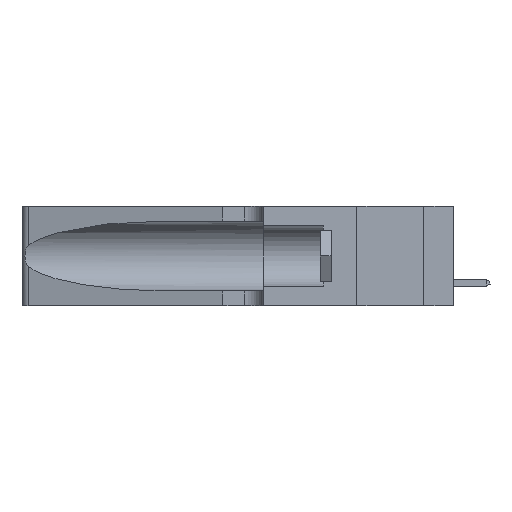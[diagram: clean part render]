
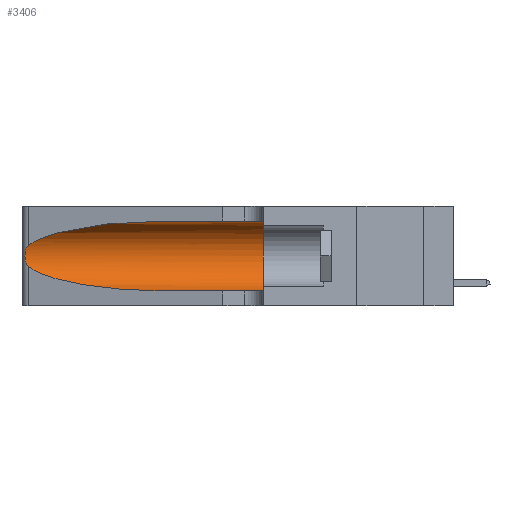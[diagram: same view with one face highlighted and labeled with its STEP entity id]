
A CAD part, left-side view. The second image highlights one B-rep face of the part: STEP entity #3406.
In plain terms, the highlighted cylindrical face has radius 3.308 mm (diameter 6.617 mm), a partial arc.
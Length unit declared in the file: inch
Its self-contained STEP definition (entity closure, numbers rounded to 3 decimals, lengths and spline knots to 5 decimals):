
#773 = DIRECTION ( 'NONE',  ( 0., 0., -1. ) ) ;
#1287 = CARTESIAN_POINT ( 'NONE',  ( 0.1305, 1.61858, 0.185 ) ) ;
#1504 = DIRECTION ( 'NONE',  ( 0., 1., 0. ) ) ;
#1772 = ORIENTED_EDGE ( 'NONE', *, *, #36571, .T. ) ;
#2330 = EDGE_CURVE ( 'NONE', #11419, #4882, #37015, .T. ) ;
#2530 = CARTESIAN_POINT ( 'NONE',  ( 0.25787, 1.23484, 0.2124 ) ) ;
#3406 = ADVANCED_FACE ( 'NONE', ( #35059 ), #34391, .F. ) ;
#4882 = VERTEX_POINT ( 'NONE', #51084 ) ;
#5034 = AXIS2_PLACEMENT_3D ( 'NONE', #48932, #1504, #29259 ) ;
#5925 = LINE ( 'NONE', #24997, #35693 ) ;
#5954 = CARTESIAN_POINT ( 'NONE',  ( 0.1305, 0.35, 0.05475 ) ) ;
#6724 = CIRCLE ( 'NONE', #5034, 0.13025 ) ;
#6942 = CARTESIAN_POINT ( 'NONE',  ( 0.25789, 1.23486, 0.15765 ) ) ;
#7525 = ORIENTED_EDGE ( 'NONE', *, *, #16669, .T. ) ;
#8419 = VERTEX_POINT ( 'NONE', #15291 ) ;
#8648 = CARTESIAN_POINT ( 'NONE',  ( 0.2373, 1.15595, 0.28018 ) ) ;
#9358 = VERTEX_POINT ( 'NONE', #5954 ) ;
#10707 = CARTESIAN_POINT ( 'NONE',  ( 0.26075, 1.23896, 0.19203 ) ) ;
#11419 = VERTEX_POINT ( 'NONE', #11508 ) ;
#11508 = CARTESIAN_POINT ( 'NONE',  ( 0.1305, 0.72297, 0.31525 ) ) ;
#11758 = CARTESIAN_POINT ( 'NONE',  ( 0.1305, 0.72297, 0.05475 ) ) ;
#12000 = VECTOR ( 'NONE', #46282, 39.37008 ) ;
#13221 = EDGE_CURVE ( 'NONE', #18733, #9358, #5925, .T. ) ;
#15284 = CARTESIAN_POINT ( 'NONE',  ( 0.18966, 0.96281, 0.05475 ) ) ;
#15291 = CARTESIAN_POINT ( 'NONE',  ( 0.25487, 1.22718, 0.14631 ) ) ;
#16669 = EDGE_CURVE ( 'NONE', #4882, #8419, #50766, .T. ) ;
#17367 = EDGE_CURVE ( 'NONE', #23731, #9358, #6724, .T. ) ;
#18733 = VERTEX_POINT ( 'NONE', #11758 ) ;
#20065 = CARTESIAN_POINT ( 'NONE',  ( 0.1305, 1.61858, 0.31525 ) ) ;
#22287 = CARTESIAN_POINT ( 'NONE',  ( 0.25639, 1.23184, 0.21858 ) ) ;
#22631 = CARTESIAN_POINT ( 'NONE',  ( 0.26075, 1.23896, 0.178 ) ) ;
#23715 = ORIENTED_EDGE ( 'NONE', *, *, #2330, .T. ) ;
#23731 = VERTEX_POINT ( 'NONE', #34816 ) ;
#24167 = ORIENTED_EDGE ( 'NONE', *, *, #13221, .T. ) ;
#24209 = CARTESIAN_POINT ( 'NONE',  ( 0.18966, 0.96281, 0.31525 ) ) ;
#24997 = CARTESIAN_POINT ( 'NONE',  ( 0.1305, 1.61858, 0.05475 ) ) ;
#26633 = CARTESIAN_POINT ( 'NONE',  ( 0.25856, 1.23593, 0.16098 ) ) ;
#29259 = DIRECTION ( 'NONE',  ( 0., 0., 1. ) ) ;
#29900 = DIRECTION ( 'NONE',  ( 0., -1., 0. ) ) ;
#30049 = CARTESIAN_POINT ( 'NONE',  ( 0.25487, 1.22718, 0.22369 ) ) ;
#30255 = CARTESIAN_POINT ( 'NONE',  ( 0.25854, 1.2359, 0.20912 ) ) ;
#32325 = EDGE_CURVE ( 'NONE', #11419, #23731, #47311, .T. ) ;
#32343 = CARTESIAN_POINT ( 'NONE',  ( 0.1305, 0.72297, 0.31525 ) ) ;
#33664 = CARTESIAN_POINT ( 'NONE',  ( 0.25555, 1.22994, 0.2215 ) ) ;
#34219 = CARTESIAN_POINT ( 'NONE',  ( 0.26018, 1.23835, 0.19895 ) ) ;
#34265 = CARTESIAN_POINT ( 'NONE',  ( 0.25555, 1.22993, 0.14849 ) ) ;
#34391 = CYLINDRICAL_SURFACE ( 'NONE', #40762, 0.13025 ) ;
#34816 = CARTESIAN_POINT ( 'NONE',  ( 0.1305, 0.35, 0.31525 ) ) ;
#34830 = CARTESIAN_POINT ( 'NONE',  ( 0.2373, 1.15595, 0.08982 ) ) ;
#35059 = FACE_OUTER_BOUND ( 'NONE', #51047, .T. ) ;
#35349 = CARTESIAN_POINT ( 'NONE',  ( 0.25487, 1.22718, 0.14631 ) ) ;
#35693 = VECTOR ( 'NONE', #29900, 39.37008 ) ;
#36571 = EDGE_CURVE ( 'NONE', #8419, #18733, #43451, .T. ) ;
#36674 = DIRECTION ( 'NONE',  ( 0., -1., 0. ) ) ;
#37015 =( BOUNDED_CURVE ( )  B_SPLINE_CURVE ( 3, ( #32343, #24209, #8648, #47775 ),
 .UNSPECIFIED., .F., .F. ) 
 B_SPLINE_CURVE_WITH_KNOTS ( ( 4, 4 ),
 ( 1.5708, 2.84003 ),
 .UNSPECIFIED. ) 
 CURVE ( )  GEOMETRIC_REPRESENTATION_ITEM ( )  RATIONAL_B_SPLINE_CURVE ( ( 1., 0.87, 0.87, 1. ) ) 
 REPRESENTATION_ITEM ( '' )  );
#38572 = CARTESIAN_POINT ( 'NONE',  ( 0.25639, 1.23186, 0.15144 ) ) ;
#40762 = AXIS2_PLACEMENT_3D ( 'NONE', #1287, #36674, #773 ) ;
#42573 = CARTESIAN_POINT ( 'NONE',  ( 0.26017, 1.23833, 0.17102 ) ) ;
#43451 =( BOUNDED_CURVE ( )  B_SPLINE_CURVE ( 3, ( #35349, #34830, #15284, #50725 ),
 .UNSPECIFIED., .F., .F. ) 
 B_SPLINE_CURVE_WITH_KNOTS ( ( 4, 4 ),
 ( 3.44316, 4.71239 ),
 .UNSPECIFIED. ) 
 CURVE ( )  GEOMETRIC_REPRESENTATION_ITEM ( )  RATIONAL_B_SPLINE_CURVE ( ( 1., 0.87, 0.87, 1. ) ) 
 REPRESENTATION_ITEM ( '' )  );
#43476 = ORIENTED_EDGE ( 'NONE', *, *, #32325, .F. ) ;
#44283 = ORIENTED_EDGE ( 'NONE', *, *, #17367, .F. ) ;
#45654 = CARTESIAN_POINT ( 'NONE',  ( 0.25487, 1.22718, 0.14631 ) ) ;
#46282 = DIRECTION ( 'NONE',  ( 0., -1., 0. ) ) ;
#47311 = LINE ( 'NONE', #20065, #12000 ) ;
#47775 = CARTESIAN_POINT ( 'NONE',  ( 0.25487, 1.22718, 0.22369 ) ) ;
#48932 = CARTESIAN_POINT ( 'NONE',  ( 0.1305, 0.35, 0.185 ) ) ;
#50725 = CARTESIAN_POINT ( 'NONE',  ( 0.1305, 0.72297, 0.05475 ) ) ;
#50766 = B_SPLINE_CURVE_WITH_KNOTS ( 'NONE', 3,
 ( #30049, #33664, #22287, #2530, #30255, #34219, #10707, #22631, #42573, #26633, #6942, #38572, #34265, #45654 ),
 .UNSPECIFIED., .F., .F.,
 ( 4, 2, 2, 2, 2, 2, 4 ),
 ( 0., 0.00027, 0.00053, 0.00107, 0.0016, 0.00187, 0.00214 ),
 .UNSPECIFIED. ) ;
#51047 = EDGE_LOOP ( 'NONE', ( #23715, #7525, #1772, #24167, #44283, #43476 ) ) ;
#51084 = CARTESIAN_POINT ( 'NONE',  ( 0.25487, 1.22718, 0.22369 ) ) ;
